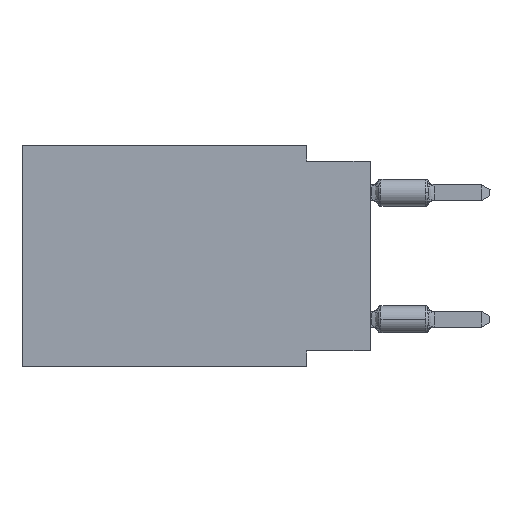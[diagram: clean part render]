
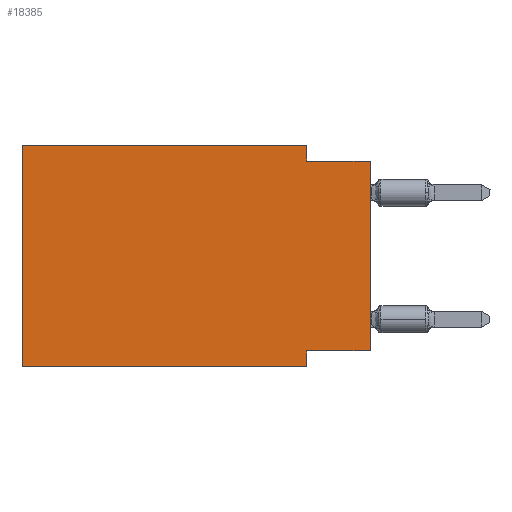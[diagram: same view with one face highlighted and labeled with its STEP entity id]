
A CAD part, left-side view. The second image highlights one B-rep face of the part: STEP entity #18385.
In plain terms, the highlighted planar face has unit normal (-1, 0, 0).
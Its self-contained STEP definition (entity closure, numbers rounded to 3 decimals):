
#1346 = EDGE_CURVE ( 'NONE', #22750, #60784, #22613, .T. ) ;
#2270 = LINE ( 'NONE', #22068, #63251 ) ;
#3632 = CARTESIAN_POINT ( 'NONE',  ( 0., 2.54, -8.255 ) ) ;
#3751 = VERTEX_POINT ( 'NONE', #15239 ) ;
#6055 = EDGE_CURVE ( 'NONE', #21939, #62384, #45629, .T. ) ;
#6836 = ORIENTED_EDGE ( 'NONE', *, *, #40333, .F. ) ;
#8033 = DIRECTION ( 'NONE',  ( 0., 0., -1. ) ) ;
#10260 = VECTOR ( 'NONE', #32003, 1000. ) ;
#10590 = CARTESIAN_POINT ( 'NONE',  ( 0., 13.97, 0. ) ) ;
#13295 = LINE ( 'NONE', #43443, #45518 ) ;
#14826 = DIRECTION ( 'NONE',  ( 1., 0., 0. ) ) ;
#15239 = CARTESIAN_POINT ( 'NONE',  ( 0., 2.54, -8.89 ) ) ;
#15712 = CARTESIAN_POINT ( 'NONE',  ( 0., 13.97, -8.89 ) ) ;
#16131 = CARTESIAN_POINT ( 'NONE',  ( 0., 0., -8.255 ) ) ;
#16761 = EDGE_LOOP ( 'NONE', ( #61167, #58164, #6836, #32725, #60990, #24914, #45925, #20717 ) ) ;
#17205 = VERTEX_POINT ( 'NONE', #29399 ) ;
#18057 = DIRECTION ( 'NONE',  ( 0., -1., 0. ) ) ;
#18385 = ADVANCED_FACE ( 'NONE', ( #44344 ), #26072, .F. ) ;
#20717 = ORIENTED_EDGE ( 'NONE', *, *, #6055, .F. ) ;
#21939 = VERTEX_POINT ( 'NONE', #57653 ) ;
#21991 = CARTESIAN_POINT ( 'NONE',  ( 0., 2.54, -8.89 ) ) ;
#22068 = CARTESIAN_POINT ( 'NONE',  ( 0., 2.54, 0. ) ) ;
#22613 = LINE ( 'NONE', #52445, #41959 ) ;
#22750 = VERTEX_POINT ( 'NONE', #46789 ) ;
#24914 = ORIENTED_EDGE ( 'NONE', *, *, #24946, .T. ) ;
#24946 = EDGE_CURVE ( 'NONE', #42768, #3751, #52852, .T. ) ;
#26059 = CARTESIAN_POINT ( 'NONE',  ( 0., 0., -0.635 ) ) ;
#26072 = PLANE ( 'NONE',  #28249 ) ;
#26854 = LINE ( 'NONE', #21991, #62154 ) ;
#27000 = VERTEX_POINT ( 'NONE', #53247 ) ;
#28249 = AXIS2_PLACEMENT_3D ( 'NONE', #44645, #14826, #54382 ) ;
#28679 = CARTESIAN_POINT ( 'NONE',  ( 0., 2.54, 0. ) ) ;
#29399 = CARTESIAN_POINT ( 'NONE',  ( 0., 0., -0.635 ) ) ;
#30062 = LINE ( 'NONE', #10590, #54329 ) ;
#31227 = DIRECTION ( 'NONE',  ( 0., -1., 0. ) ) ;
#32003 = DIRECTION ( 'NONE',  ( 0., 1., 0. ) ) ;
#32725 = ORIENTED_EDGE ( 'NONE', *, *, #1346, .F. ) ;
#38142 = EDGE_CURVE ( 'NONE', #62384, #3751, #26854, .T. ) ;
#39202 = EDGE_CURVE ( 'NONE', #21939, #17205, #13295, .T. ) ;
#40123 = DIRECTION ( 'NONE',  ( 0., 0., 1. ) ) ;
#40333 = EDGE_CURVE ( 'NONE', #60784, #27000, #2270, .T. ) ;
#41226 = DIRECTION ( 'NONE',  ( 0., 0., -1. ) ) ;
#41884 = VECTOR ( 'NONE', #31227, 1000. ) ;
#41959 = VECTOR ( 'NONE', #18057, 1000. ) ;
#42265 = LINE ( 'NONE', #26059, #41884 ) ;
#42768 = VERTEX_POINT ( 'NONE', #15712 ) ;
#43125 = EDGE_CURVE ( 'NONE', #42768, #22750, #30062, .T. ) ;
#43142 = DIRECTION ( 'NONE',  ( 0., -1., 0. ) ) ;
#43443 = CARTESIAN_POINT ( 'NONE',  ( 0., 0., 0. ) ) ;
#44344 = FACE_OUTER_BOUND ( 'NONE', #16761, .T. ) ;
#44645 = CARTESIAN_POINT ( 'NONE',  ( 0., 13.97, 0. ) ) ;
#45518 = VECTOR ( 'NONE', #47356, 1000. ) ;
#45629 = LINE ( 'NONE', #16131, #10260 ) ;
#45925 = ORIENTED_EDGE ( 'NONE', *, *, #38142, .F. ) ;
#46789 = CARTESIAN_POINT ( 'NONE',  ( 0., 13.97, 0. ) ) ;
#47356 = DIRECTION ( 'NONE',  ( 0., 0., 1. ) ) ;
#47975 = CARTESIAN_POINT ( 'NONE',  ( 0., 13.97, -8.89 ) ) ;
#52445 = CARTESIAN_POINT ( 'NONE',  ( 0., 13.97, 0. ) ) ;
#52852 = LINE ( 'NONE', #47975, #62549 ) ;
#53247 = CARTESIAN_POINT ( 'NONE',  ( 0., 2.54, -0.635 ) ) ;
#54329 = VECTOR ( 'NONE', #40123, 1000. ) ;
#54382 = DIRECTION ( 'NONE',  ( 0., 0., -1. ) ) ;
#57653 = CARTESIAN_POINT ( 'NONE',  ( 0., 0., -8.255 ) ) ;
#58164 = ORIENTED_EDGE ( 'NONE', *, *, #62227, .F. ) ;
#60784 = VERTEX_POINT ( 'NONE', #28679 ) ;
#60990 = ORIENTED_EDGE ( 'NONE', *, *, #43125, .F. ) ;
#61167 = ORIENTED_EDGE ( 'NONE', *, *, #39202, .T. ) ;
#62154 = VECTOR ( 'NONE', #8033, 1000. ) ;
#62227 = EDGE_CURVE ( 'NONE', #27000, #17205, #42265, .T. ) ;
#62384 = VERTEX_POINT ( 'NONE', #3632 ) ;
#62549 = VECTOR ( 'NONE', #43142, 1000. ) ;
#63251 = VECTOR ( 'NONE', #41226, 1000. ) ;
